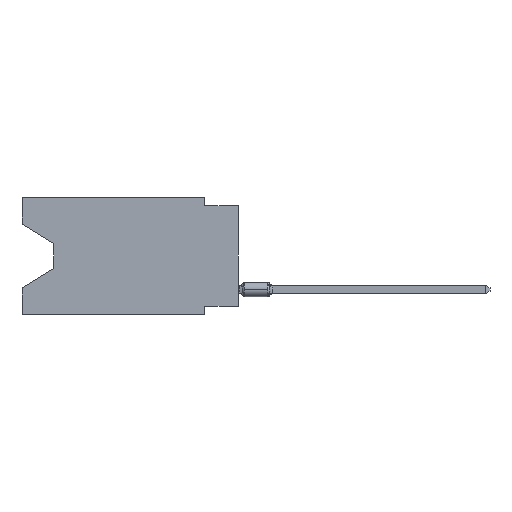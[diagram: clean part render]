
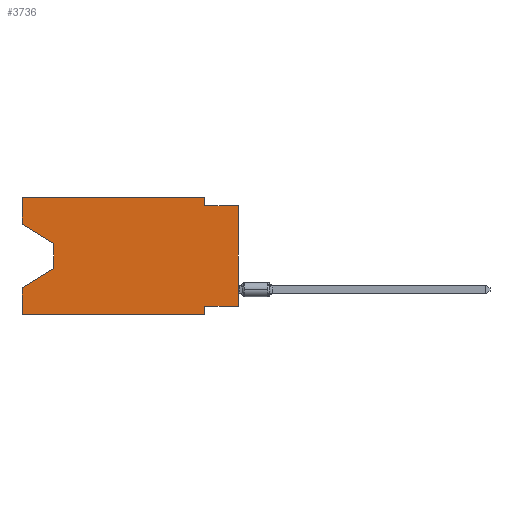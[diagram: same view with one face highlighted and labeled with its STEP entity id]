
A CAD part, left-side view. The second image highlights one B-rep face of the part: STEP entity #3736.
In plain terms, the highlighted planar face has unit normal (-1, 0, 0).
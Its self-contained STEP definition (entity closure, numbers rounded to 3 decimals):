
#56 = DIRECTION ( 'NONE',  ( 0., 0., 1. ) ) ;
#61 = ORIENTED_EDGE ( 'NONE', *, *, #8359, .F. ) ;
#281 = CARTESIAN_POINT ( 'NONE',  ( 0., 13.97, -3.505 ) ) ;
#525 = DIRECTION ( 'NONE',  ( 0., -1., 0. ) ) ;
#569 = FACE_OUTER_BOUND ( 'NONE', #14066, .T. ) ;
#1054 = VERTEX_POINT ( 'NONE', #3746 ) ;
#1063 = LINE ( 'NONE', #6905, #4101 ) ;
#1159 = DIRECTION ( 'NONE',  ( 0., 0., 1. ) ) ;
#1490 = LINE ( 'NONE', #10531, #10857 ) ;
#1491 = CARTESIAN_POINT ( 'NONE',  ( 0., 16.383, -8.89 ) ) ;
#1518 = CARTESIAN_POINT ( 'NONE',  ( 0., 0., -8.255 ) ) ;
#1568 = CARTESIAN_POINT ( 'NONE',  ( 0., 16.383, -8.89 ) ) ;
#1755 = LINE ( 'NONE', #3045, #5242 ) ;
#1910 = DIRECTION ( 'NONE',  ( 0., -1., 0. ) ) ;
#2200 = EDGE_CURVE ( 'NONE', #3149, #10958, #1755, .T. ) ;
#2253 = LINE ( 'NONE', #15030, #5596 ) ;
#2779 = LINE ( 'NONE', #3015, #11674 ) ;
#2911 = DIRECTION ( 'NONE',  ( 0., 0.855, -0.519 ) ) ;
#3015 = CARTESIAN_POINT ( 'NONE',  ( 0., 16.383, 0. ) ) ;
#3045 = CARTESIAN_POINT ( 'NONE',  ( 0., 0., -0.635 ) ) ;
#3068 = ORIENTED_EDGE ( 'NONE', *, *, #2200, .F. ) ;
#3149 = VERTEX_POINT ( 'NONE', #14893 ) ;
#3265 = VERTEX_POINT ( 'NONE', #12968 ) ;
#3352 = VECTOR ( 'NONE', #14410, 1000. ) ;
#3556 = CARTESIAN_POINT ( 'NONE',  ( 0., 0., -0.635 ) ) ;
#3650 = VERTEX_POINT ( 'NONE', #13944 ) ;
#3676 = ORIENTED_EDGE ( 'NONE', *, *, #11396, .F. ) ;
#3736 = ADVANCED_FACE ( 'NONE', ( #569 ), #3842, .F. ) ;
#3746 = CARTESIAN_POINT ( 'NONE',  ( 0., 2.54, -8.255 ) ) ;
#3779 = LINE ( 'NONE', #1568, #13831 ) ;
#3842 = PLANE ( 'NONE',  #5983 ) ;
#4014 = VERTEX_POINT ( 'NONE', #8062 ) ;
#4048 = EDGE_CURVE ( 'NONE', #10748, #10958, #13860, .T. ) ;
#4101 = VECTOR ( 'NONE', #14682, 1000. ) ;
#4251 = CARTESIAN_POINT ( 'NONE',  ( 0., 2.54, -8.89 ) ) ;
#4329 = VECTOR ( 'NONE', #2911, 1000. ) ;
#4398 = VERTEX_POINT ( 'NONE', #4251 ) ;
#4448 = DIRECTION ( 'NONE',  ( 0., -0.855, -0.519 ) ) ;
#4749 = DIRECTION ( 'NONE',  ( 0., 0., 1. ) ) ;
#4908 = DIRECTION ( 'NONE',  ( 0., 0., -1. ) ) ;
#5242 = VECTOR ( 'NONE', #1910, 1000. ) ;
#5354 = LINE ( 'NONE', #10915, #3352 ) ;
#5596 = VECTOR ( 'NONE', #56, 1000. ) ;
#5871 = CARTESIAN_POINT ( 'NONE',  ( 0., 0., 0. ) ) ;
#5983 = AXIS2_PLACEMENT_3D ( 'NONE', #9602, #13110, #6113 ) ;
#6113 = DIRECTION ( 'NONE',  ( 0., 0., -1. ) ) ;
#6124 = EDGE_CURVE ( 'NONE', #3265, #13045, #2779, .T. ) ;
#6236 = VERTEX_POINT ( 'NONE', #15019 ) ;
#6905 = CARTESIAN_POINT ( 'NONE',  ( 0., 0., -8.255 ) ) ;
#7082 = ORIENTED_EDGE ( 'NONE', *, *, #13784, .F. ) ;
#7112 = ORIENTED_EDGE ( 'NONE', *, *, #4048, .T. ) ;
#7404 = LINE ( 'NONE', #281, #13286 ) ;
#7435 = VECTOR ( 'NONE', #1159, 1000. ) ;
#7489 = EDGE_CURVE ( 'NONE', #10903, #4014, #13722, .T. ) ;
#7787 = VECTOR ( 'NONE', #4448, 1000. ) ;
#7988 = EDGE_CURVE ( 'NONE', #13045, #3149, #8223, .T. ) ;
#8062 = CARTESIAN_POINT ( 'NONE',  ( 0., 13.97, -3.505 ) ) ;
#8191 = EDGE_CURVE ( 'NONE', #3650, #6236, #13323, .T. ) ;
#8223 = LINE ( 'NONE', #13007, #13799 ) ;
#8359 = EDGE_CURVE ( 'NONE', #10748, #1054, #1063, .T. ) ;
#8443 = ORIENTED_EDGE ( 'NONE', *, *, #9013, .T. ) ;
#9013 = EDGE_CURVE ( 'NONE', #12636, #4398, #3779, .T. ) ;
#9157 = CARTESIAN_POINT ( 'NONE',  ( 0., 16.383, -2.038 ) ) ;
#9498 = ORIENTED_EDGE ( 'NONE', *, *, #8191, .T. ) ;
#9602 = CARTESIAN_POINT ( 'NONE',  ( 0., 16.383, 0. ) ) ;
#10006 = DIRECTION ( 'NONE',  ( 0., -1., 0. ) ) ;
#10476 = EDGE_CURVE ( 'NONE', #1054, #4398, #5354, .T. ) ;
#10531 = CARTESIAN_POINT ( 'NONE',  ( 0., 16.383, 0. ) ) ;
#10748 = VERTEX_POINT ( 'NONE', #1518 ) ;
#10806 = DIRECTION ( 'NONE',  ( 0., 0., -1. ) ) ;
#10857 = VECTOR ( 'NONE', #4749, 1000. ) ;
#10903 = VERTEX_POINT ( 'NONE', #12744 ) ;
#10915 = CARTESIAN_POINT ( 'NONE',  ( 0., 2.54, -8.89 ) ) ;
#10953 = ORIENTED_EDGE ( 'NONE', *, *, #7988, .F. ) ;
#10958 = VERTEX_POINT ( 'NONE', #3556 ) ;
#11342 = ORIENTED_EDGE ( 'NONE', *, *, #7489, .T. ) ;
#11396 = EDGE_CURVE ( 'NONE', #10903, #3265, #2253, .T. ) ;
#11674 = VECTOR ( 'NONE', #10006, 1000. ) ;
#11696 = ORIENTED_EDGE ( 'NONE', *, *, #6124, .F. ) ;
#11709 = ORIENTED_EDGE ( 'NONE', *, *, #10476, .F. ) ;
#12100 = CARTESIAN_POINT ( 'NONE',  ( 0., 13.97, -5.385 ) ) ;
#12636 = VERTEX_POINT ( 'NONE', #1491 ) ;
#12744 = CARTESIAN_POINT ( 'NONE',  ( 0., 16.383, -2.038 ) ) ;
#12968 = CARTESIAN_POINT ( 'NONE',  ( 0., 16.383, 0. ) ) ;
#13007 = CARTESIAN_POINT ( 'NONE',  ( 0., 2.54, 0. ) ) ;
#13045 = VERTEX_POINT ( 'NONE', #14550 ) ;
#13110 = DIRECTION ( 'NONE',  ( 1., 0., 0. ) ) ;
#13187 = ORIENTED_EDGE ( 'NONE', *, *, #13875, .T. ) ;
#13286 = VECTOR ( 'NONE', #4908, 1000. ) ;
#13323 = LINE ( 'NONE', #12100, #4329 ) ;
#13722 = LINE ( 'NONE', #9157, #7787 ) ;
#13784 = EDGE_CURVE ( 'NONE', #12636, #6236, #1490, .T. ) ;
#13799 = VECTOR ( 'NONE', #10806, 1000. ) ;
#13831 = VECTOR ( 'NONE', #525, 1000. ) ;
#13860 = LINE ( 'NONE', #5871, #7435 ) ;
#13875 = EDGE_CURVE ( 'NONE', #4014, #3650, #7404, .T. ) ;
#13944 = CARTESIAN_POINT ( 'NONE',  ( 0., 13.97, -5.385 ) ) ;
#14066 = EDGE_LOOP ( 'NONE', ( #11342, #13187, #9498, #7082, #8443, #11709, #61, #7112, #3068, #10953, #11696, #3676 ) ) ;
#14410 = DIRECTION ( 'NONE',  ( 0., 0., -1. ) ) ;
#14550 = CARTESIAN_POINT ( 'NONE',  ( 0., 2.54, 0. ) ) ;
#14682 = DIRECTION ( 'NONE',  ( 0., 1., 0. ) ) ;
#14893 = CARTESIAN_POINT ( 'NONE',  ( 0., 2.54, -0.635 ) ) ;
#15019 = CARTESIAN_POINT ( 'NONE',  ( 0., 16.383, -6.852 ) ) ;
#15030 = CARTESIAN_POINT ( 'NONE',  ( 0., 16.383, 0. ) ) ;
